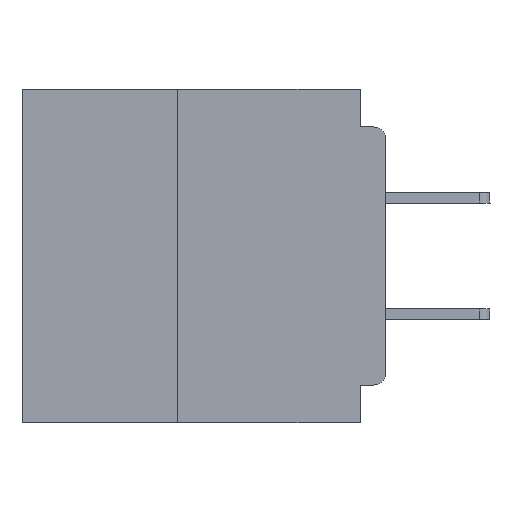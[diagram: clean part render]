
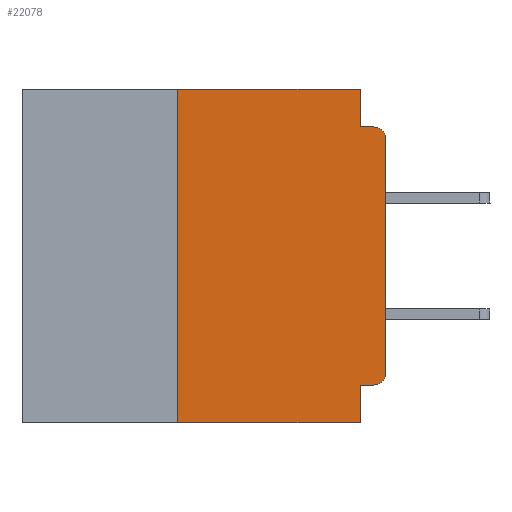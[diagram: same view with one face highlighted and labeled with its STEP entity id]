
A CAD part, left-side view. The second image highlights one B-rep face of the part: STEP entity #22078.
In plain terms, the highlighted planar face has unit normal (-1, 0, 0).
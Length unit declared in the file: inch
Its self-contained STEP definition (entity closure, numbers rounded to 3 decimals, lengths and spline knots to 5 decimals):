
#1251 = ORIENTED_EDGE ( 'NONE', *, *, #13144, .F. ) ;
#1268 = DIRECTION ( 'NONE',  ( 0., 0., -1. ) ) ;
#1508 = DIRECTION ( 'NONE',  ( 0., 0., -1. ) ) ;
#1766 = CARTESIAN_POINT ( 'NONE',  ( 0., 0.437, -0.4 ) ) ;
#2878 = VECTOR ( 'NONE', #12282, 39.37008 ) ;
#3339 = DIRECTION ( 'NONE',  ( 0., 0., 1. ) ) ;
#6203 = CARTESIAN_POINT ( 'NONE',  ( 0., 0.437, 0. ) ) ;
#6209 = EDGE_CURVE ( 'NONE', #62535, #15601, #22838, .T. ) ;
#6379 = EDGE_CURVE ( 'NONE', #13576, #24031, #52862, .T. ) ;
#7475 = AXIS2_PLACEMENT_3D ( 'NONE', #6203, #11477, #47860 ) ;
#8224 = LINE ( 'NONE', #37788, #49742 ) ;
#11477 = DIRECTION ( 'NONE',  ( 1., 0., 0. ) ) ;
#12103 = VERTEX_POINT ( 'NONE', #16213 ) ;
#12282 = DIRECTION ( 'NONE',  ( 0., -1., 0. ) ) ;
#13144 = EDGE_CURVE ( 'NONE', #15601, #39518, #45753, .T. ) ;
#13576 = VERTEX_POINT ( 'NONE', #65994 ) ;
#15135 = CARTESIAN_POINT ( 'NONE',  ( 0., 0.25, 0. ) ) ;
#15168 = VECTOR ( 'NONE', #60739, 39.37008 ) ;
#15601 = VERTEX_POINT ( 'NONE', #15135 ) ;
#15793 = EDGE_CURVE ( 'NONE', #24031, #48807, #21018, .T. ) ;
#15876 = ORIENTED_EDGE ( 'NONE', *, *, #25442, .T. ) ;
#16213 = CARTESIAN_POINT ( 'NONE',  ( 0., 0.015, -0.355 ) ) ;
#16693 = CARTESIAN_POINT ( 'NONE',  ( 0., 0.015, -0.06 ) ) ;
#16919 = DIRECTION ( 'NONE',  ( 0., 1., 0. ) ) ;
#17849 = FACE_OUTER_BOUND ( 'NONE', #44108, .T. ) ;
#18282 = ORIENTED_EDGE ( 'NONE', *, *, #66284, .F. ) ;
#20217 = CARTESIAN_POINT ( 'NONE',  ( 0., 0.437, 0. ) ) ;
#21018 = CIRCLE ( 'NONE', #28536, 0.015 ) ;
#21594 = CIRCLE ( 'NONE', #33171, 0.015 ) ;
#21958 = DIRECTION ( 'NONE',  ( 0., 0., -1. ) ) ;
#22078 = ADVANCED_FACE ( 'NONE', ( #17849 ), #37436, .F. ) ;
#22171 = CARTESIAN_POINT ( 'NONE',  ( 0., 0., -0.355 ) ) ;
#22838 = LINE ( 'NONE', #48652, #50451 ) ;
#24031 = VERTEX_POINT ( 'NONE', #27637 ) ;
#24399 = CARTESIAN_POINT ( 'NONE',  ( 0., 0.031, 0. ) ) ;
#25016 = CARTESIAN_POINT ( 'NONE',  ( 0., 0.031, -0.045 ) ) ;
#25129 = ORIENTED_EDGE ( 'NONE', *, *, #6379, .T. ) ;
#25442 = EDGE_CURVE ( 'NONE', #62535, #44705, #44442, .T. ) ;
#26788 = ORIENTED_EDGE ( 'NONE', *, *, #60999, .F. ) ;
#27637 = CARTESIAN_POINT ( 'NONE',  ( 0., 0., -0.06 ) ) ;
#28536 = AXIS2_PLACEMENT_3D ( 'NONE', #16693, #53048, #21958 ) ;
#30641 = EDGE_CURVE ( 'NONE', #12103, #42405, #63300, .T. ) ;
#30888 = CARTESIAN_POINT ( 'NONE',  ( 0., 0.031, -0.355 ) ) ;
#32471 = DIRECTION ( 'NONE',  ( -1., 0., 0. ) ) ;
#32795 = ORIENTED_EDGE ( 'NONE', *, *, #30641, .F. ) ;
#33171 = AXIS2_PLACEMENT_3D ( 'NONE', #63611, #32471, #1268 ) ;
#33198 = DIRECTION ( 'NONE',  ( 0., 0., 1. ) ) ;
#33893 = ORIENTED_EDGE ( 'NONE', *, *, #53997, .T. ) ;
#34323 = CARTESIAN_POINT ( 'NONE',  ( 0., 0., 0. ) ) ;
#35691 = VECTOR ( 'NONE', #16919, 39.37008 ) ;
#37436 = PLANE ( 'NONE',  #7475 ) ;
#37788 = CARTESIAN_POINT ( 'NONE',  ( 0., 0., -0.045 ) ) ;
#37925 = ORIENTED_EDGE ( 'NONE', *, *, #6209, .F. ) ;
#39055 = VECTOR ( 'NONE', #3339, 39.37008 ) ;
#39518 = VERTEX_POINT ( 'NONE', #39670 ) ;
#39670 = CARTESIAN_POINT ( 'NONE',  ( 0., 0.031, 0. ) ) ;
#40159 = VECTOR ( 'NONE', #1508, 39.37008 ) ;
#42405 = VERTEX_POINT ( 'NONE', #30888 ) ;
#44108 = EDGE_LOOP ( 'NONE', ( #25129, #67111, #26788, #58219, #1251, #37925, #15876, #18282, #32795, #33893 ) ) ;
#44424 = LINE ( 'NONE', #24399, #15168 ) ;
#44442 = LINE ( 'NONE', #1766, #2878 ) ;
#44705 = VERTEX_POINT ( 'NONE', #45381 ) ;
#45381 = CARTESIAN_POINT ( 'NONE',  ( 0., 0.031, -0.4 ) ) ;
#45753 = LINE ( 'NONE', #20217, #61206 ) ;
#47860 = DIRECTION ( 'NONE',  ( 0., 0., -1. ) ) ;
#48390 = CARTESIAN_POINT ( 'NONE',  ( 0., 0.031, -0.4 ) ) ;
#48652 = CARTESIAN_POINT ( 'NONE',  ( 0., 0.25, -0.4 ) ) ;
#48807 = VERTEX_POINT ( 'NONE', #59340 ) ;
#49742 = VECTOR ( 'NONE', #58431, 39.37008 ) ;
#50451 = VECTOR ( 'NONE', #33198, 39.37008 ) ;
#52862 = LINE ( 'NONE', #34323, #39055 ) ;
#53048 = DIRECTION ( 'NONE',  ( -1., 0., 0. ) ) ;
#53971 = LINE ( 'NONE', #48390, #40159 ) ;
#53997 = EDGE_CURVE ( 'NONE', #12103, #13576, #21594, .T. ) ;
#58219 = ORIENTED_EDGE ( 'NONE', *, *, #64801, .F. ) ;
#58431 = DIRECTION ( 'NONE',  ( 0., -1., 0. ) ) ;
#59340 = CARTESIAN_POINT ( 'NONE',  ( 0., 0.015, -0.045 ) ) ;
#59412 = VERTEX_POINT ( 'NONE', #25016 ) ;
#60739 = DIRECTION ( 'NONE',  ( 0., 0., -1. ) ) ;
#60999 = EDGE_CURVE ( 'NONE', #59412, #48807, #8224, .T. ) ;
#61206 = VECTOR ( 'NONE', #66949, 39.37008 ) ;
#61673 = CARTESIAN_POINT ( 'NONE',  ( 0., 0.25, -0.4 ) ) ;
#62535 = VERTEX_POINT ( 'NONE', #61673 ) ;
#63300 = LINE ( 'NONE', #22171, #35691 ) ;
#63611 = CARTESIAN_POINT ( 'NONE',  ( 0., 0.015, -0.34 ) ) ;
#64801 = EDGE_CURVE ( 'NONE', #39518, #59412, #44424, .T. ) ;
#65994 = CARTESIAN_POINT ( 'NONE',  ( 0., 0., -0.34 ) ) ;
#66284 = EDGE_CURVE ( 'NONE', #42405, #44705, #53971, .T. ) ;
#66949 = DIRECTION ( 'NONE',  ( 0., -1., 0. ) ) ;
#67111 = ORIENTED_EDGE ( 'NONE', *, *, #15793, .T. ) ;
